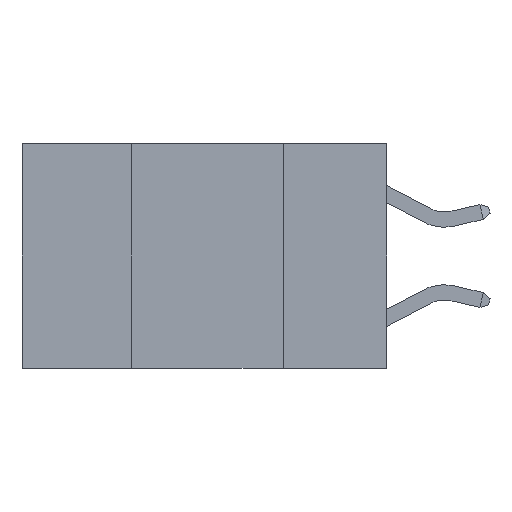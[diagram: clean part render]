
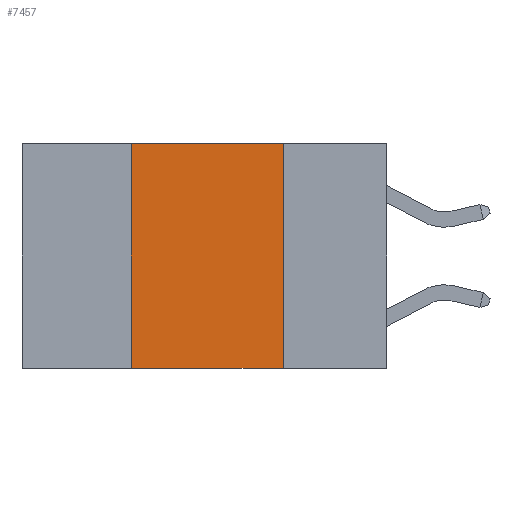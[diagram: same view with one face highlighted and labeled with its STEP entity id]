
A CAD part, left-side view. The second image highlights one B-rep face of the part: STEP entity #7457.
In plain terms, the highlighted planar face has unit normal (-1, 0, 0).
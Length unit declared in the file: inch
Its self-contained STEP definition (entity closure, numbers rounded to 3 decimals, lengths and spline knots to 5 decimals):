
#15 = LINE ( 'NONE', #12352, #5465 ) ;
#167 = CARTESIAN_POINT ( 'NONE',  ( 0., 0.17, 0. ) ) ;
#679 = EDGE_CURVE ( 'NONE', #10656, #12952, #4775, .T. ) ;
#1359 = ORIENTED_EDGE ( 'NONE', *, *, #679, .F. ) ;
#2083 = CARTESIAN_POINT ( 'NONE',  ( 0., 0.42, -0.37 ) ) ;
#2319 = DIRECTION ( 'NONE',  ( 0., -1., 0. ) ) ;
#3393 = PLANE ( 'NONE',  #7343 ) ;
#3575 = ORIENTED_EDGE ( 'NONE', *, *, #13355, .F. ) ;
#3751 = DIRECTION ( 'NONE',  ( 0., 0., 1. ) ) ;
#4106 = EDGE_CURVE ( 'NONE', #10656, #6566, #15, .T. ) ;
#4183 = EDGE_LOOP ( 'NONE', ( #6758, #3575, #1359, #7132 ) ) ;
#4568 = CARTESIAN_POINT ( 'NONE',  ( 0., 0.42, 0. ) ) ;
#4775 = LINE ( 'NONE', #4568, #8109 ) ;
#4978 = CARTESIAN_POINT ( 'NONE',  ( 0., 0.17, -0.37 ) ) ;
#5195 = CARTESIAN_POINT ( 'NONE',  ( 0., 0.17, 0. ) ) ;
#5465 = VECTOR ( 'NONE', #6183, 39.37008 ) ;
#6183 = DIRECTION ( 'NONE',  ( 0., -1., 0. ) ) ;
#6283 = VECTOR ( 'NONE', #10608, 39.37008 ) ;
#6566 = VERTEX_POINT ( 'NONE', #4978 ) ;
#6758 = ORIENTED_EDGE ( 'NONE', *, *, #9333, .F. ) ;
#6995 = CARTESIAN_POINT ( 'NONE',  ( 0., 0.42, 0. ) ) ;
#7132 = ORIENTED_EDGE ( 'NONE', *, *, #4106, .T. ) ;
#7343 = AXIS2_PLACEMENT_3D ( 'NONE', #12495, #9305, #11024 ) ;
#7457 = ADVANCED_FACE ( 'NONE', ( #8574 ), #3393, .F. ) ;
#7583 = LINE ( 'NONE', #8596, #9994 ) ;
#8109 = VECTOR ( 'NONE', #3751, 39.37008 ) ;
#8574 = FACE_OUTER_BOUND ( 'NONE', #4183, .T. ) ;
#8596 = CARTESIAN_POINT ( 'NONE',  ( 0., 0.6, 0. ) ) ;
#8930 = VERTEX_POINT ( 'NONE', #167 ) ;
#9305 = DIRECTION ( 'NONE',  ( 1., 0., 0. ) ) ;
#9333 = EDGE_CURVE ( 'NONE', #8930, #6566, #11614, .T. ) ;
#9994 = VECTOR ( 'NONE', #2319, 39.37008 ) ;
#10608 = DIRECTION ( 'NONE',  ( 0., 0., -1. ) ) ;
#10656 = VERTEX_POINT ( 'NONE', #2083 ) ;
#11024 = DIRECTION ( 'NONE',  ( 0., 0., -1. ) ) ;
#11614 = LINE ( 'NONE', #5195, #6283 ) ;
#12352 = CARTESIAN_POINT ( 'NONE',  ( 0., 0.6, -0.37 ) ) ;
#12495 = CARTESIAN_POINT ( 'NONE',  ( 0., 0.6, 0. ) ) ;
#12952 = VERTEX_POINT ( 'NONE', #6995 ) ;
#13355 = EDGE_CURVE ( 'NONE', #12952, #8930, #7583, .T. ) ;
